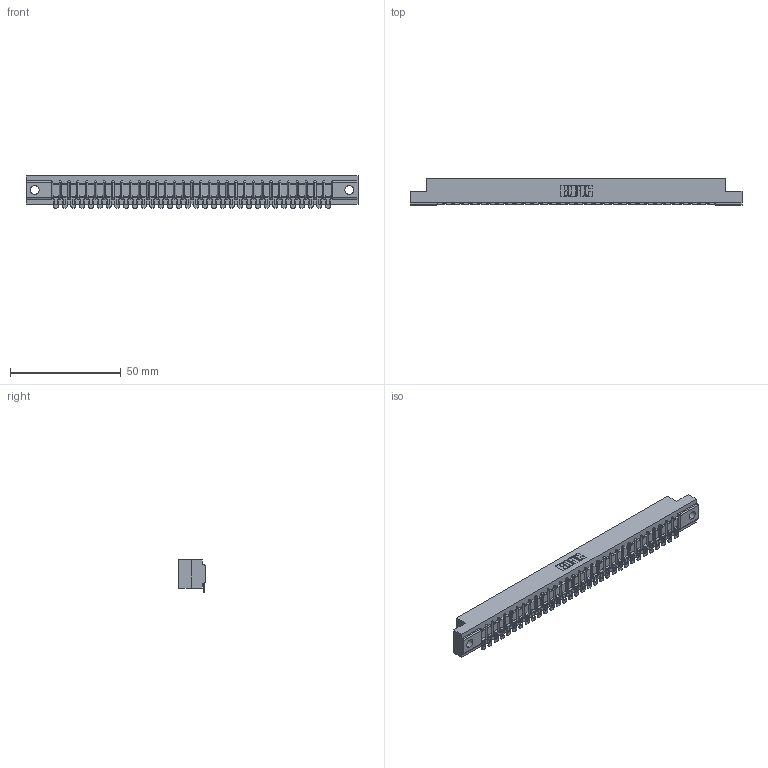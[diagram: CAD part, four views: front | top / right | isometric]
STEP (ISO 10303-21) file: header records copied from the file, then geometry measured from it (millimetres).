
FILE_DESCRIPTION (( 'STEP AP203' ), '1' );
FILE_NAME ('357-032-454-104.STEP', '2020-10-02T06:17:12', ( '' ), ( '' ), 'SwSTEP 2.0', 'SolidWorks 2020', '' );
FILE_SCHEMA (( 'CONFIG_CONTROL_DESIGN' ));
Length unit declared in the file: inch
Products named in the file (3): 357-032-454-104; 307-290-002_554; 307 Part_.156 Dia Mounting Holes
Assembly tree (33 placements, depth 2):
  357-032-454-104
    307 Part_.156 Dia Mounting Holes
    307-290-002_554  x32
Bounding box: 149.81 x 12.01 x 14.52 mm (x, y, z)
Volume: 15862.5 mm3; surface area: 19685 mm2
Topology: 33 solids, 33 shells, 2757 faces, 8455 edges, 5546 vertices
Faces by surface type: plane 1556, cylinder 1135, sphere 66
Entity records: 30049 total; most frequent: CARTESIAN_POINT 5072, ORIENTED_EDGE 5060, DIRECTION 4930, EDGE_CURVE 2530, VECTOR 1934, LINE 1934, VERTEX_POINT 1640, AXIS2_PLACEMENT_3D 1498
